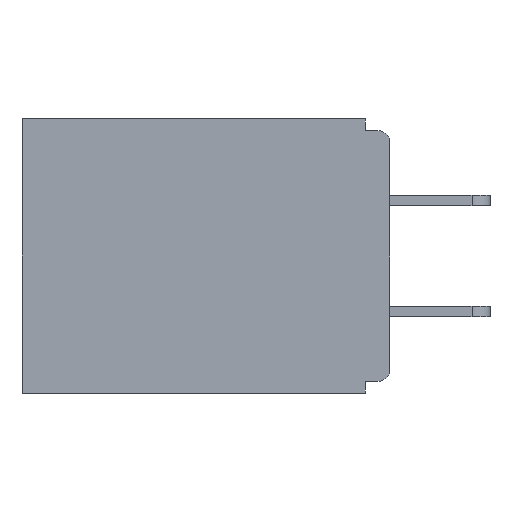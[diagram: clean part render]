
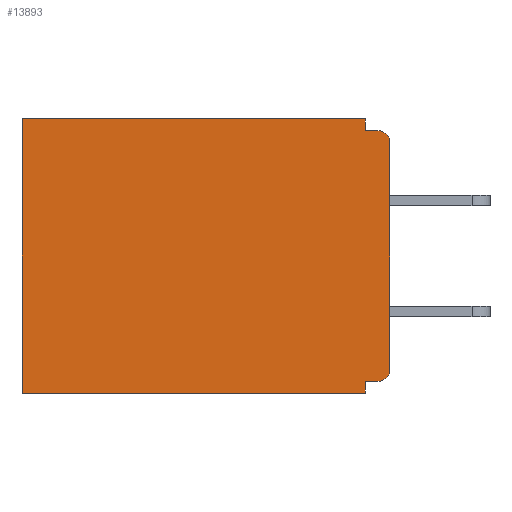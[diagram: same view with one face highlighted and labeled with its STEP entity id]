
A CAD part, left-side view. The second image highlights one B-rep face of the part: STEP entity #13893.
In plain terms, the highlighted planar face has unit normal (-1, 0, 0).
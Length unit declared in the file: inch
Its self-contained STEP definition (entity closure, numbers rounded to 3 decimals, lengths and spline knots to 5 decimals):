
#147 = CARTESIAN_POINT ( 'NONE',  ( 0.298, 0., -0.343 ) ) ;
#170 = DIRECTION ( 'NONE',  ( 0., 0., -1. ) ) ;
#408 = EDGE_CURVE ( 'NONE', #11657, #2357, #13188, .T. ) ;
#621 = DIRECTION ( 'NONE',  ( 0., 0., -1. ) ) ;
#847 = PLANE ( 'NONE',  #8994 ) ;
#894 = VERTEX_POINT ( 'NONE', #2217 ) ;
#956 = VECTOR ( 'NONE', #10813, 39.37008 ) ;
#1016 = VERTEX_POINT ( 'NONE', #14176 ) ;
#1346 = EDGE_CURVE ( 'NONE', #3685, #5633, #11121, .T. ) ;
#1593 = CARTESIAN_POINT ( 'NONE',  ( 0.298, 0.46, 0. ) ) ;
#1782 = VECTOR ( 'NONE', #170, 39.37008 ) ;
#1859 = DIRECTION ( 'NONE',  ( -1., 0., 0. ) ) ;
#2217 = CARTESIAN_POINT ( 'NONE',  ( 0.298, 0., -0.313 ) ) ;
#2357 = VERTEX_POINT ( 'NONE', #14339 ) ;
#2359 = CARTESIAN_POINT ( 'NONE',  ( 0.298, 0.015, -0.03 ) ) ;
#2501 = ORIENTED_EDGE ( 'NONE', *, *, #10597, .F. ) ;
#2714 = FACE_OUTER_BOUND ( 'NONE', #12483, .T. ) ;
#3207 = CARTESIAN_POINT ( 'NONE',  ( 0.298, 0., 0. ) ) ;
#3480 = CARTESIAN_POINT ( 'NONE',  ( 0.298, 0.015, -0.015 ) ) ;
#3544 = VERTEX_POINT ( 'NONE', #12357 ) ;
#3685 = VERTEX_POINT ( 'NONE', #12927 ) ;
#4152 = DIRECTION ( 'NONE',  ( 0., 0., -1. ) ) ;
#4314 = CARTESIAN_POINT ( 'NONE',  ( 0.298, 0.031, -0.343 ) ) ;
#4682 = VECTOR ( 'NONE', #6591, 39.37008 ) ;
#4942 = LINE ( 'NONE', #6270, #14916 ) ;
#5099 = VERTEX_POINT ( 'NONE', #5151 ) ;
#5151 = CARTESIAN_POINT ( 'NONE',  ( 0.298, 0., -0.03 ) ) ;
#5633 = VERTEX_POINT ( 'NONE', #6017 ) ;
#5836 = VECTOR ( 'NONE', #14602, 39.37008 ) ;
#5967 = DIRECTION ( 'NONE',  ( 0., 0., -1. ) ) ;
#6017 = CARTESIAN_POINT ( 'NONE',  ( 0.298, 0.031, -0.343 ) ) ;
#6201 = LINE ( 'NONE', #8419, #1782 ) ;
#6270 = CARTESIAN_POINT ( 'NONE',  ( 0.298, 0., -0.328 ) ) ;
#6591 = DIRECTION ( 'NONE',  ( 0., 1., 0. ) ) ;
#6643 = ORIENTED_EDGE ( 'NONE', *, *, #8945, .T. ) ;
#6644 = DIRECTION ( 'NONE',  ( 0., 0., -1. ) ) ;
#6700 = VERTEX_POINT ( 'NONE', #10331 ) ;
#6703 = ORIENTED_EDGE ( 'NONE', *, *, #7013, .F. ) ;
#6791 = VERTEX_POINT ( 'NONE', #3480 ) ;
#6801 = CIRCLE ( 'NONE', #8821, 0.015 ) ;
#6918 = ORIENTED_EDGE ( 'NONE', *, *, #408, .T. ) ;
#7013 = EDGE_CURVE ( 'NONE', #5633, #6700, #7818, .T. ) ;
#7125 = DIRECTION ( 'NONE',  ( -1., 0., 0. ) ) ;
#7191 = DIRECTION ( 'NONE',  ( 0., -1., 0. ) ) ;
#7340 = AXIS2_PLACEMENT_3D ( 'NONE', #2359, #7125, #5967 ) ;
#7576 = LINE ( 'NONE', #7708, #13423 ) ;
#7625 = ORIENTED_EDGE ( 'NONE', *, *, #13676, .F. ) ;
#7708 = CARTESIAN_POINT ( 'NONE',  ( 0.298, 0., 0. ) ) ;
#7818 = LINE ( 'NONE', #147, #956 ) ;
#8208 = ORIENTED_EDGE ( 'NONE', *, *, #9282, .F. ) ;
#8419 = CARTESIAN_POINT ( 'NONE',  ( 0.298, 0.031, -0.343 ) ) ;
#8806 = CARTESIAN_POINT ( 'NONE',  ( 0.298, 0.015, -0.313 ) ) ;
#8821 = AXIS2_PLACEMENT_3D ( 'NONE', #8806, #1859, #621 ) ;
#8892 = ORIENTED_EDGE ( 'NONE', *, *, #14918, .T. ) ;
#8945 = EDGE_CURVE ( 'NONE', #1016, #894, #6801, .T. ) ;
#8994 = AXIS2_PLACEMENT_3D ( 'NONE', #3207, #11479, #15089 ) ;
#9189 = CARTESIAN_POINT ( 'NONE',  ( 0.298, 0.031, 0. ) ) ;
#9282 = EDGE_CURVE ( 'NONE', #3544, #6791, #15282, .T. ) ;
#10078 = CARTESIAN_POINT ( 'NONE',  ( 0.298, 0., 0. ) ) ;
#10331 = CARTESIAN_POINT ( 'NONE',  ( 0.298, 0.46, -0.343 ) ) ;
#10493 = EDGE_CURVE ( 'NONE', #2357, #6700, #14126, .T. ) ;
#10597 = EDGE_CURVE ( 'NONE', #11657, #3544, #6201, .T. ) ;
#10645 = CARTESIAN_POINT ( 'NONE',  ( 0.298, 0., -0.015 ) ) ;
#10775 = VECTOR ( 'NONE', #6644, 39.37008 ) ;
#10813 = DIRECTION ( 'NONE',  ( 0., 1., 0. ) ) ;
#11121 = LINE ( 'NONE', #4314, #10775 ) ;
#11162 = ORIENTED_EDGE ( 'NONE', *, *, #1346, .F. ) ;
#11203 = ORIENTED_EDGE ( 'NONE', *, *, #10493, .T. ) ;
#11354 = ORIENTED_EDGE ( 'NONE', *, *, #13851, .F. ) ;
#11479 = DIRECTION ( 'NONE',  ( 1., 0., 0. ) ) ;
#11657 = VERTEX_POINT ( 'NONE', #9189 ) ;
#12357 = CARTESIAN_POINT ( 'NONE',  ( 0.298, 0.031, -0.015 ) ) ;
#12483 = EDGE_LOOP ( 'NONE', ( #8892, #8208, #2501, #6918, #11203, #6703, #11162, #7625, #6643, #11354 ) ) ;
#12927 = CARTESIAN_POINT ( 'NONE',  ( 0.298, 0.031, -0.328 ) ) ;
#13188 = LINE ( 'NONE', #10078, #4682 ) ;
#13423 = VECTOR ( 'NONE', #4152, 39.37008 ) ;
#13676 = EDGE_CURVE ( 'NONE', #1016, #3685, #4942, .T. ) ;
#13851 = EDGE_CURVE ( 'NONE', #5099, #894, #7576, .T. ) ;
#13893 = ADVANCED_FACE ( 'NONE', ( #2714 ), #847, .F. ) ;
#14126 = LINE ( 'NONE', #1593, #5836 ) ;
#14176 = CARTESIAN_POINT ( 'NONE',  ( 0.298, 0.015, -0.328 ) ) ;
#14339 = CARTESIAN_POINT ( 'NONE',  ( 0.298, 0.46, 0. ) ) ;
#14586 = DIRECTION ( 'NONE',  ( 0., 1., 0. ) ) ;
#14602 = DIRECTION ( 'NONE',  ( 0., 0., -1. ) ) ;
#14908 = VECTOR ( 'NONE', #7191, 39.37008 ) ;
#14916 = VECTOR ( 'NONE', #14586, 39.37008 ) ;
#14918 = EDGE_CURVE ( 'NONE', #5099, #6791, #15270, .T. ) ;
#15089 = DIRECTION ( 'NONE',  ( 0., 0., -1. ) ) ;
#15270 = CIRCLE ( 'NONE', #7340, 0.015 ) ;
#15282 = LINE ( 'NONE', #10645, #14908 ) ;
